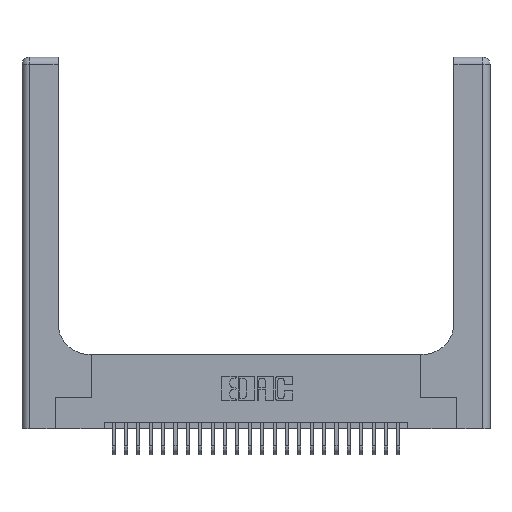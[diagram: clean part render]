
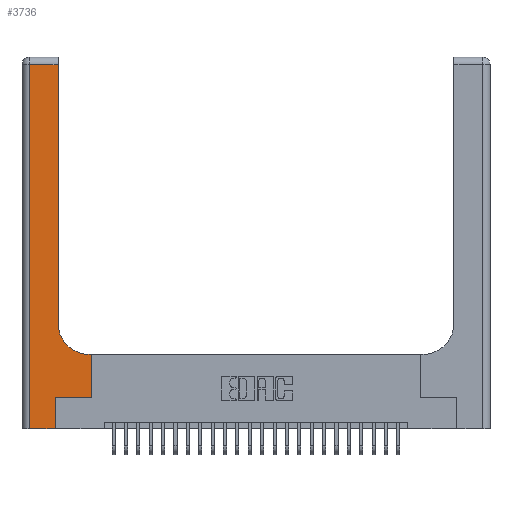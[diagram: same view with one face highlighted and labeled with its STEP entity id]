
A CAD part, top view. The second image highlights one B-rep face of the part: STEP entity #3736.
In plain terms, the highlighted planar face has unit normal (0, 0, 1).
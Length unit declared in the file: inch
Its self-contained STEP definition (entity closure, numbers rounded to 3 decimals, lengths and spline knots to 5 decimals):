
#40 = VERTEX_POINT ( 'NONE', #12633 ) ;
#215 = DIRECTION ( 'NONE',  ( -1., 0., 0. ) ) ;
#568 = CARTESIAN_POINT ( 'NONE',  ( 0., 2.94, 0.37 ) ) ;
#845 = DIRECTION ( 'NONE',  ( 0., 0., -1. ) ) ;
#1023 = VERTEX_POINT ( 'NONE', #27572 ) ;
#1383 = EDGE_CURVE ( 'NONE', #26477, #15658, #25040, .T. ) ;
#2147 = CARTESIAN_POINT ( 'NONE',  ( 0.2915, 3., 0.37 ) ) ;
#2318 = CARTESIAN_POINT ( 'NONE',  ( 0.06, 0., 0.37 ) ) ;
#2523 = DIRECTION ( 'NONE',  ( -1., 0., 0. ) ) ;
#2594 = CARTESIAN_POINT ( 'NONE',  ( 0., 0., 0.37 ) ) ;
#3141 = ORIENTED_EDGE ( 'NONE', *, *, #5753, .T. ) ;
#3280 = AXIS2_PLACEMENT_3D ( 'NONE', #15669, #8928, #215 ) ;
#3494 = VECTOR ( 'NONE', #24081, 39.37008 ) ;
#3561 = VECTOR ( 'NONE', #25214, 39.37008 ) ;
#3736 = ADVANCED_FACE ( 'NONE', ( #18166 ), #21743, .F. ) ;
#4478 = EDGE_CURVE ( 'NONE', #15658, #23620, #8580, .T. ) ;
#5467 = DIRECTION ( 'NONE',  ( 1., 0., 0. ) ) ;
#5595 = CARTESIAN_POINT ( 'NONE',  ( 0.5585, 0.25, 0.37 ) ) ;
#5753 = EDGE_CURVE ( 'NONE', #7208, #1023, #9320, .T. ) ;
#5838 = EDGE_CURVE ( 'NONE', #23341, #12848, #27255, .T. ) ;
#7061 = DIRECTION ( 'NONE',  ( 1., 0., 0. ) ) ;
#7196 = CARTESIAN_POINT ( 'NONE',  ( 0.2915, 0.6, 0.37 ) ) ;
#7208 = VERTEX_POINT ( 'NONE', #24851 ) ;
#7668 = VECTOR ( 'NONE', #17315, 39.37008 ) ;
#7832 = CARTESIAN_POINT ( 'NONE',  ( 0.5585, 0.6, 0.37 ) ) ;
#8552 = ORIENTED_EDGE ( 'NONE', *, *, #25956, .T. ) ;
#8580 = LINE ( 'NONE', #23901, #3494 ) ;
#8595 = AXIS2_PLACEMENT_3D ( 'NONE', #24705, #845, #5467 ) ;
#8928 = DIRECTION ( 'NONE',  ( 0., 0., -1. ) ) ;
#9320 = LINE ( 'NONE', #10402, #3561 ) ;
#10402 = CARTESIAN_POINT ( 'NONE',  ( 0.269, 0., 0.37 ) ) ;
#10585 = CARTESIAN_POINT ( 'NONE',  ( 0.06, 2.94, 0.37 ) ) ;
#10753 = VECTOR ( 'NONE', #16116, 39.37008 ) ;
#12633 = CARTESIAN_POINT ( 'NONE',  ( 0.2915, 0.85, 0.37 ) ) ;
#12806 = CARTESIAN_POINT ( 'NONE',  ( 0.2915, 2.94, 0.37 ) ) ;
#12848 = VERTEX_POINT ( 'NONE', #7832 ) ;
#13932 = EDGE_CURVE ( 'NONE', #40, #26477, #15161, .T. ) ;
#15161 = LINE ( 'NONE', #2147, #24643 ) ;
#15457 = EDGE_CURVE ( 'NONE', #12848, #23457, #22874, .T. ) ;
#15658 = VERTEX_POINT ( 'NONE', #10585 ) ;
#15669 = CARTESIAN_POINT ( 'NONE',  ( 0., 3., 0.37 ) ) ;
#15926 = ORIENTED_EDGE ( 'NONE', *, *, #5838, .T. ) ;
#15928 = EDGE_CURVE ( 'NONE', #23620, #7208, #19748, .T. ) ;
#16116 = DIRECTION ( 'NONE',  ( -1., 0., 0. ) ) ;
#16500 = ORIENTED_EDGE ( 'NONE', *, *, #1383, .T. ) ;
#17315 = DIRECTION ( 'NONE',  ( 1., 0., 0. ) ) ;
#17783 = ORIENTED_EDGE ( 'NONE', *, *, #15457, .T. ) ;
#17914 = CIRCLE ( 'NONE', #8595, 0.25 ) ;
#18115 = EDGE_CURVE ( 'NONE', #23457, #40, #17914, .T. ) ;
#18150 = VECTOR ( 'NONE', #27079, 39.37008 ) ;
#18166 = FACE_OUTER_BOUND ( 'NONE', #20638, .T. ) ;
#18569 = LINE ( 'NONE', #21634, #7668 ) ;
#19106 = ORIENTED_EDGE ( 'NONE', *, *, #15928, .T. ) ;
#19748 = LINE ( 'NONE', #2594, #23534 ) ;
#20638 = EDGE_LOOP ( 'NONE', ( #24746, #16500, #23737, #19106, #3141, #8552, #15926, #17783, #26101 ) ) ;
#21340 = DIRECTION ( 'NONE',  ( 0., 1., 0. ) ) ;
#21634 = CARTESIAN_POINT ( 'NONE',  ( 0.269, 0.25, 0.37 ) ) ;
#21743 = PLANE ( 'NONE',  #3280 ) ;
#22874 = LINE ( 'NONE', #7196, #27557 ) ;
#23341 = VERTEX_POINT ( 'NONE', #5595 ) ;
#23457 = VERTEX_POINT ( 'NONE', #25780 ) ;
#23534 = VECTOR ( 'NONE', #7061, 39.37008 ) ;
#23620 = VERTEX_POINT ( 'NONE', #2318 ) ;
#23737 = ORIENTED_EDGE ( 'NONE', *, *, #4478, .T. ) ;
#23901 = CARTESIAN_POINT ( 'NONE',  ( 0.06, 3., 0.37 ) ) ;
#24081 = DIRECTION ( 'NONE',  ( 0., -1., 0. ) ) ;
#24643 = VECTOR ( 'NONE', #21340, 39.37008 ) ;
#24705 = CARTESIAN_POINT ( 'NONE',  ( 0.5415, 0.85, 0.37 ) ) ;
#24746 = ORIENTED_EDGE ( 'NONE', *, *, #13932, .T. ) ;
#24851 = CARTESIAN_POINT ( 'NONE',  ( 0.269, 0., 0.37 ) ) ;
#25040 = LINE ( 'NONE', #568, #10753 ) ;
#25214 = DIRECTION ( 'NONE',  ( 0., 1., 0. ) ) ;
#25780 = CARTESIAN_POINT ( 'NONE',  ( 0.5415, 0.6, 0.37 ) ) ;
#25956 = EDGE_CURVE ( 'NONE', #1023, #23341, #18569, .T. ) ;
#26101 = ORIENTED_EDGE ( 'NONE', *, *, #18115, .T. ) ;
#26477 = VERTEX_POINT ( 'NONE', #12806 ) ;
#26979 = CARTESIAN_POINT ( 'NONE',  ( 0.5585, 0.25, 0.37 ) ) ;
#27079 = DIRECTION ( 'NONE',  ( 0., 1., 0. ) ) ;
#27255 = LINE ( 'NONE', #26979, #18150 ) ;
#27557 = VECTOR ( 'NONE', #2523, 39.37008 ) ;
#27572 = CARTESIAN_POINT ( 'NONE',  ( 0.269, 0.25, 0.37 ) ) ;
